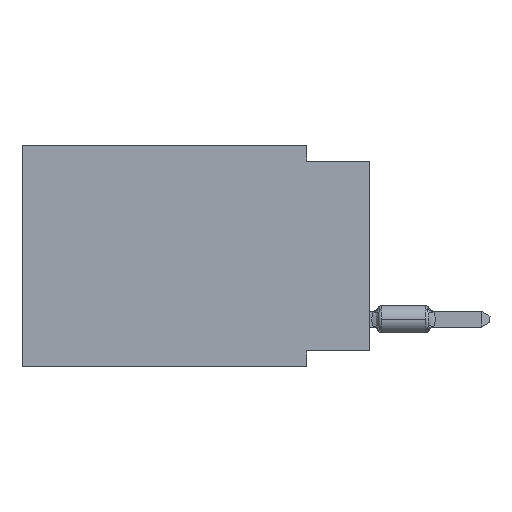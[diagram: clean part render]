
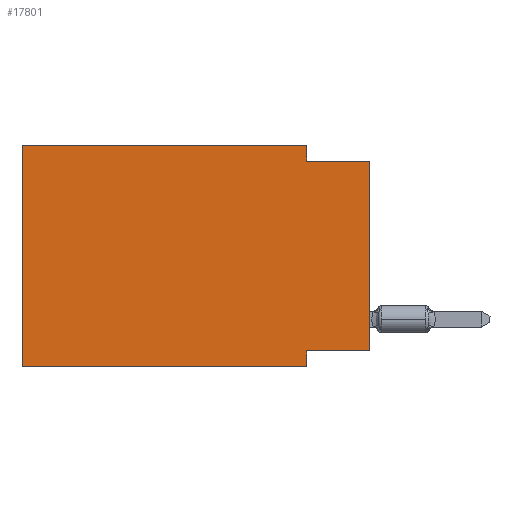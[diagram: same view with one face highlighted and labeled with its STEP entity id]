
A CAD part, left-side view. The second image highlights one B-rep face of the part: STEP entity #17801.
In plain terms, the highlighted planar face has unit normal (-1, 0, 0).
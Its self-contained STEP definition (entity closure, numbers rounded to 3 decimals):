
#93 = VERTEX_POINT ( 'NONE', #15004 ) ;
#95 = VECTOR ( 'NONE', #11106, 1000. ) ;
#909 = VECTOR ( 'NONE', #16632, 1000. ) ;
#1425 = LINE ( 'NONE', #19265, #17408 ) ;
#2362 = PLANE ( 'NONE',  #18575 ) ;
#2411 = ORIENTED_EDGE ( 'NONE', *, *, #14028, .T. ) ;
#2767 = VERTEX_POINT ( 'NONE', #19393 ) ;
#3194 = VERTEX_POINT ( 'NONE', #15918 ) ;
#3210 = EDGE_CURVE ( 'NONE', #2767, #20413, #1425, .T. ) ;
#3939 = CARTESIAN_POINT ( 'NONE',  ( 0., 13.97, 0. ) ) ;
#4040 = LINE ( 'NONE', #3939, #909 ) ;
#4047 = EDGE_CURVE ( 'NONE', #3194, #10437, #6861, .T. ) ;
#6087 = VECTOR ( 'NONE', #12892, 1000. ) ;
#6209 = VERTEX_POINT ( 'NONE', #10919 ) ;
#6505 = ORIENTED_EDGE ( 'NONE', *, *, #4047, .F. ) ;
#6547 = LINE ( 'NONE', #7136, #6087 ) ;
#6861 = LINE ( 'NONE', #19646, #12020 ) ;
#7097 = DIRECTION ( 'NONE',  ( 0., 0., -1. ) ) ;
#7136 = CARTESIAN_POINT ( 'NONE',  ( 0., 0., 0. ) ) ;
#7323 = VECTOR ( 'NONE', #7097, 1000. ) ;
#7628 = CARTESIAN_POINT ( 'NONE',  ( 0., 0., -0.635 ) ) ;
#7767 = CARTESIAN_POINT ( 'NONE',  ( 0., 2.54, 0. ) ) ;
#8213 = DIRECTION ( 'NONE',  ( 0., -1., 0. ) ) ;
#8272 = VERTEX_POINT ( 'NONE', #19970 ) ;
#8377 = ORIENTED_EDGE ( 'NONE', *, *, #3210, .F. ) ;
#8547 = DIRECTION ( 'NONE',  ( 0., -1., 0. ) ) ;
#8860 = VECTOR ( 'NONE', #8213, 1000. ) ;
#9044 = VECTOR ( 'NONE', #9374, 1000. ) ;
#9089 = ORIENTED_EDGE ( 'NONE', *, *, #10563, .F. ) ;
#9374 = DIRECTION ( 'NONE',  ( 0., 0., -1. ) ) ;
#9386 = EDGE_CURVE ( 'NONE', #10437, #2767, #13451, .T. ) ;
#9415 = ORIENTED_EDGE ( 'NONE', *, *, #19354, .F. ) ;
#10437 = VERTEX_POINT ( 'NONE', #7767 ) ;
#10563 = EDGE_CURVE ( 'NONE', #14912, #3194, #4040, .T. ) ;
#10641 = ORIENTED_EDGE ( 'NONE', *, *, #12508, .F. ) ;
#10919 = CARTESIAN_POINT ( 'NONE',  ( 0., 0., -8.255 ) ) ;
#10990 = ORIENTED_EDGE ( 'NONE', *, *, #9386, .F. ) ;
#11106 = DIRECTION ( 'NONE',  ( 0., 1., 0. ) ) ;
#11243 = DIRECTION ( 'NONE',  ( 0., -1., 0. ) ) ;
#12020 = VECTOR ( 'NONE', #8547, 1000. ) ;
#12087 = DIRECTION ( 'NONE',  ( 1., 0., 0. ) ) ;
#12237 = LINE ( 'NONE', #12548, #9044 ) ;
#12508 = EDGE_CURVE ( 'NONE', #8272, #93, #12237, .T. ) ;
#12548 = CARTESIAN_POINT ( 'NONE',  ( 0., 2.54, -8.89 ) ) ;
#12892 = DIRECTION ( 'NONE',  ( 0., 0., 1. ) ) ;
#13144 = CARTESIAN_POINT ( 'NONE',  ( 0., 13.97, -8.89 ) ) ;
#13451 = LINE ( 'NONE', #19673, #7323 ) ;
#14028 = EDGE_CURVE ( 'NONE', #14912, #93, #19406, .T. ) ;
#14607 = CARTESIAN_POINT ( 'NONE',  ( 0., 0., -8.255 ) ) ;
#14912 = VERTEX_POINT ( 'NONE', #13144 ) ;
#15004 = CARTESIAN_POINT ( 'NONE',  ( 0., 2.54, -8.89 ) ) ;
#15384 = DIRECTION ( 'NONE',  ( 0., 0., -1. ) ) ;
#15918 = CARTESIAN_POINT ( 'NONE',  ( 0., 13.97, 0. ) ) ;
#16098 = LINE ( 'NONE', #14607, #95 ) ;
#16263 = CARTESIAN_POINT ( 'NONE',  ( 0., 13.97, -8.89 ) ) ;
#16632 = DIRECTION ( 'NONE',  ( 0., 0., 1. ) ) ;
#17180 = EDGE_CURVE ( 'NONE', #6209, #20413, #6547, .T. ) ;
#17259 = FACE_OUTER_BOUND ( 'NONE', #19110, .T. ) ;
#17408 = VECTOR ( 'NONE', #11243, 1000. ) ;
#17801 = ADVANCED_FACE ( 'NONE', ( #17259 ), #2362, .F. ) ;
#18575 = AXIS2_PLACEMENT_3D ( 'NONE', #20102, #12087, #15384 ) ;
#19110 = EDGE_LOOP ( 'NONE', ( #20744, #8377, #10990, #6505, #9089, #2411, #10641, #9415 ) ) ;
#19265 = CARTESIAN_POINT ( 'NONE',  ( 0., 0., -0.635 ) ) ;
#19354 = EDGE_CURVE ( 'NONE', #6209, #8272, #16098, .T. ) ;
#19393 = CARTESIAN_POINT ( 'NONE',  ( 0., 2.54, -0.635 ) ) ;
#19406 = LINE ( 'NONE', #16263, #8860 ) ;
#19646 = CARTESIAN_POINT ( 'NONE',  ( 0., 13.97, 0. ) ) ;
#19673 = CARTESIAN_POINT ( 'NONE',  ( 0., 2.54, 0. ) ) ;
#19970 = CARTESIAN_POINT ( 'NONE',  ( 0., 2.54, -8.255 ) ) ;
#20102 = CARTESIAN_POINT ( 'NONE',  ( 0., 13.97, 0. ) ) ;
#20413 = VERTEX_POINT ( 'NONE', #7628 ) ;
#20744 = ORIENTED_EDGE ( 'NONE', *, *, #17180, .T. ) ;
